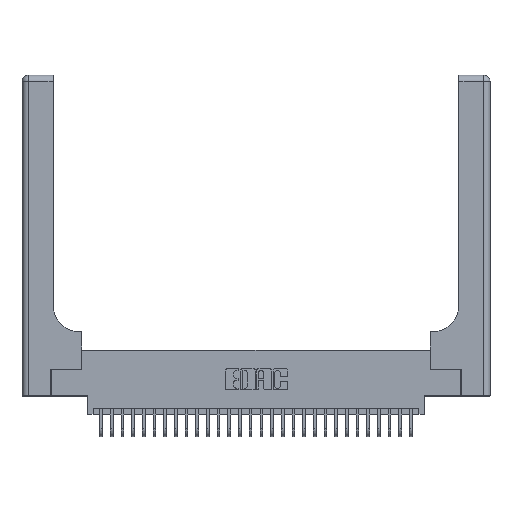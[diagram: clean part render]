
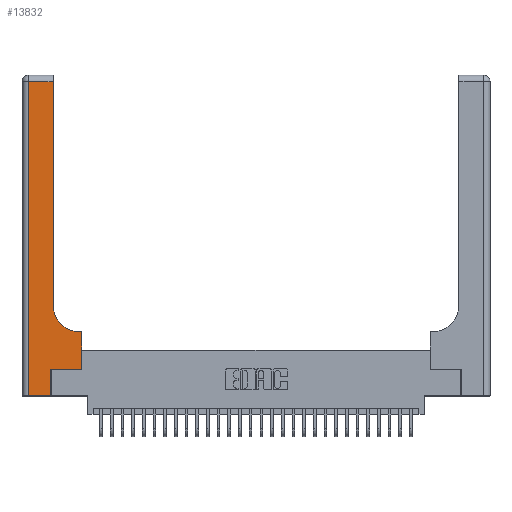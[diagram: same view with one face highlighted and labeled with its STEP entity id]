
A CAD part, top view. The second image highlights one B-rep face of the part: STEP entity #13832.
In plain terms, the highlighted planar face has unit normal (0, 0, 1).
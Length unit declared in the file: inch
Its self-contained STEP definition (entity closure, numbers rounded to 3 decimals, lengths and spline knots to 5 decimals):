
#143 = LINE ( 'NONE', #30150, #18434 ) ;
#1141 = VECTOR ( 'NONE', #6444, 39.37008 ) ;
#2508 = VECTOR ( 'NONE', #7658, 39.37008 ) ;
#2816 = DIRECTION ( 'NONE',  ( 0., -1., 0. ) ) ;
#3437 = ORIENTED_EDGE ( 'NONE', *, *, #18055, .T. ) ;
#4381 = DIRECTION ( 'NONE',  ( 0., 0., -1. ) ) ;
#4482 = CARTESIAN_POINT ( 'NONE',  ( 0.06, 0., 0.37 ) ) ;
#4663 = ORIENTED_EDGE ( 'NONE', *, *, #5269, .T. ) ;
#4709 = ORIENTED_EDGE ( 'NONE', *, *, #10287, .T. ) ;
#4841 = VECTOR ( 'NONE', #8972, 39.37008 ) ;
#4904 = VERTEX_POINT ( 'NONE', #21039 ) ;
#4951 = VERTEX_POINT ( 'NONE', #8721 ) ;
#5269 = EDGE_CURVE ( 'NONE', #28302, #21206, #24680, .T. ) ;
#5982 = EDGE_CURVE ( 'NONE', #4904, #19372, #18411, .T. ) ;
#6114 = CARTESIAN_POINT ( 'NONE',  ( 0.2915, 0.85, 0.37 ) ) ;
#6129 = VECTOR ( 'NONE', #16700, 39.37008 ) ;
#6444 = DIRECTION ( 'NONE',  ( 0., 1., 0. ) ) ;
#6706 = PLANE ( 'NONE',  #26442 ) ;
#7658 = DIRECTION ( 'NONE',  ( 1., 0., 0. ) ) ;
#7791 = EDGE_CURVE ( 'NONE', #21206, #23482, #20241, .T. ) ;
#7926 = DIRECTION ( 'NONE',  ( -1., 0., 0. ) ) ;
#8391 = ORIENTED_EDGE ( 'NONE', *, *, #16117, .T. ) ;
#8721 = CARTESIAN_POINT ( 'NONE',  ( 0.06, 2.94, 0.37 ) ) ;
#8972 = DIRECTION ( 'NONE',  ( 1., 0., 0. ) ) ;
#9638 = LINE ( 'NONE', #15681, #22130 ) ;
#10287 = EDGE_CURVE ( 'NONE', #4951, #27738, #143, .T. ) ;
#10373 = FACE_OUTER_BOUND ( 'NONE', #11038, .T. ) ;
#11038 = EDGE_LOOP ( 'NONE', ( #8391, #16394, #4709, #21125, #28131, #4663, #14077, #3437, #14642 ) ) ;
#11947 = CARTESIAN_POINT ( 'NONE',  ( 0.269, 0.25, 0.37 ) ) ;
#13158 = CARTESIAN_POINT ( 'NONE',  ( 0.2915, 2.94, 0.37 ) ) ;
#13223 = AXIS2_PLACEMENT_3D ( 'NONE', #19304, #4381, #21785 ) ;
#13351 = CARTESIAN_POINT ( 'NONE',  ( 0.269, 0., 0.37 ) ) ;
#13832 = ADVANCED_FACE ( 'NONE', ( #10373 ), #6706, .F. ) ;
#14077 = ORIENTED_EDGE ( 'NONE', *, *, #7791, .T. ) ;
#14178 = CARTESIAN_POINT ( 'NONE',  ( 0.269, 0., 0.37 ) ) ;
#14206 = CARTESIAN_POINT ( 'NONE',  ( 0., 3., 0.37 ) ) ;
#14642 = ORIENTED_EDGE ( 'NONE', *, *, #5982, .T. ) ;
#15681 = CARTESIAN_POINT ( 'NONE',  ( 0., 2.94, 0.37 ) ) ;
#16117 = EDGE_CURVE ( 'NONE', #19372, #29899, #31006, .T. ) ;
#16394 = ORIENTED_EDGE ( 'NONE', *, *, #16682, .T. ) ;
#16682 = EDGE_CURVE ( 'NONE', #29899, #4951, #9638, .T. ) ;
#16700 = DIRECTION ( 'NONE',  ( 0., 1., 0. ) ) ;
#16729 = DIRECTION ( 'NONE',  ( -1., 0., 0. ) ) ;
#16998 = EDGE_CURVE ( 'NONE', #28146, #28302, #19400, .T. ) ;
#17588 = CARTESIAN_POINT ( 'NONE',  ( 0., 0., 0.37 ) ) ;
#18055 = EDGE_CURVE ( 'NONE', #23482, #4904, #25887, .T. ) ;
#18212 = DIRECTION ( 'NONE',  ( -1., 0., 0. ) ) ;
#18411 = CIRCLE ( 'NONE', #13223, 0.25 ) ;
#18434 = VECTOR ( 'NONE', #2816, 39.37008 ) ;
#19304 = CARTESIAN_POINT ( 'NONE',  ( 0.5415, 0.85, 0.37 ) ) ;
#19372 = VERTEX_POINT ( 'NONE', #6114 ) ;
#19400 = LINE ( 'NONE', #14178, #6129 ) ;
#20241 = LINE ( 'NONE', #21357, #1141 ) ;
#20505 = DIRECTION ( 'NONE',  ( 0., 1., 0. ) ) ;
#21039 = CARTESIAN_POINT ( 'NONE',  ( 0.5415, 0.6, 0.37 ) ) ;
#21125 = ORIENTED_EDGE ( 'NONE', *, *, #27215, .T. ) ;
#21206 = VERTEX_POINT ( 'NONE', #21770 ) ;
#21357 = CARTESIAN_POINT ( 'NONE',  ( 0.5585, 0.25, 0.37 ) ) ;
#21770 = CARTESIAN_POINT ( 'NONE',  ( 0.5585, 0.25, 0.37 ) ) ;
#21785 = DIRECTION ( 'NONE',  ( 1., 0., 0. ) ) ;
#22130 = VECTOR ( 'NONE', #18212, 39.37008 ) ;
#23482 = VERTEX_POINT ( 'NONE', #27539 ) ;
#23570 = VECTOR ( 'NONE', #7926, 39.37008 ) ;
#23879 = CARTESIAN_POINT ( 'NONE',  ( 0.269, 0.25, 0.37 ) ) ;
#24680 = LINE ( 'NONE', #23879, #4841 ) ;
#24693 = LINE ( 'NONE', #17588, #2508 ) ;
#25253 = VECTOR ( 'NONE', #20505, 39.37008 ) ;
#25316 = CARTESIAN_POINT ( 'NONE',  ( 0.2915, 0.6, 0.37 ) ) ;
#25887 = LINE ( 'NONE', #25316, #23570 ) ;
#26442 = AXIS2_PLACEMENT_3D ( 'NONE', #14206, #31538, #16729 ) ;
#27215 = EDGE_CURVE ( 'NONE', #27738, #28146, #24693, .T. ) ;
#27539 = CARTESIAN_POINT ( 'NONE',  ( 0.5585, 0.6, 0.37 ) ) ;
#27738 = VERTEX_POINT ( 'NONE', #4482 ) ;
#28131 = ORIENTED_EDGE ( 'NONE', *, *, #16998, .T. ) ;
#28146 = VERTEX_POINT ( 'NONE', #13351 ) ;
#28302 = VERTEX_POINT ( 'NONE', #11947 ) ;
#29899 = VERTEX_POINT ( 'NONE', #13158 ) ;
#30150 = CARTESIAN_POINT ( 'NONE',  ( 0.06, 3., 0.37 ) ) ;
#30322 = CARTESIAN_POINT ( 'NONE',  ( 0.2915, 3., 0.37 ) ) ;
#31006 = LINE ( 'NONE', #30322, #25253 ) ;
#31538 = DIRECTION ( 'NONE',  ( 0., 0., -1. ) ) ;
